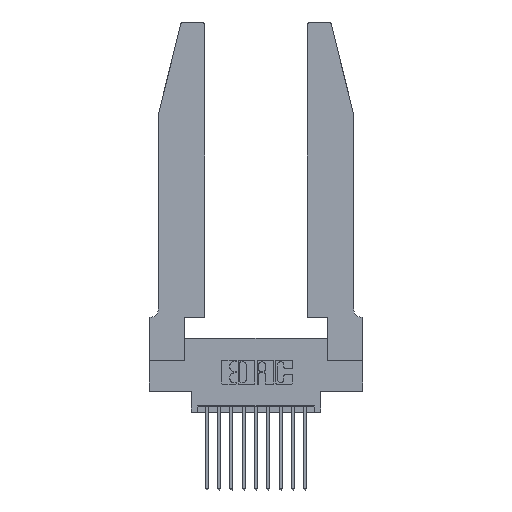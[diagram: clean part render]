
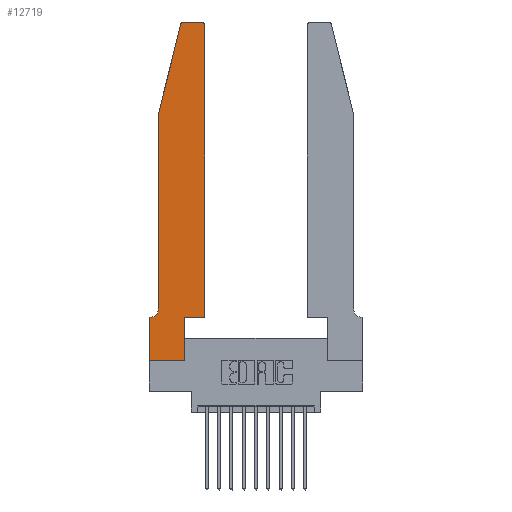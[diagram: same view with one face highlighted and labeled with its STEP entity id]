
A CAD part, top view. The second image highlights one B-rep face of the part: STEP entity #12719.
In plain terms, the highlighted planar face has unit normal (0, 0, 1).
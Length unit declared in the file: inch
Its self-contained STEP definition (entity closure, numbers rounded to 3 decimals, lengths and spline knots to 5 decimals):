
#7 = VERTEX_POINT ( 'NONE', #5723 ) ;
#8 = ORIENTED_EDGE ( 'NONE', *, *, #6700, .T. ) ;
#240 = VECTOR ( 'NONE', #7956, 39.37008 ) ;
#513 = EDGE_CURVE ( 'NONE', #15229, #9144, #12579, .T. ) ;
#574 = CARTESIAN_POINT ( 'NONE',  ( 0.0755, 2., 0.37 ) ) ;
#583 = DIRECTION ( 'NONE',  ( 0., -1., 0. ) ) ;
#691 = EDGE_CURVE ( 'NONE', #2168, #7, #15413, .T. ) ;
#982 = CARTESIAN_POINT ( 'NONE',  ( 0.2865, 0.35, 0.37 ) ) ;
#1098 = CARTESIAN_POINT ( 'NONE',  ( 0.0755, 2., 0.37 ) ) ;
#1359 = VERTEX_POINT ( 'NONE', #3333 ) ;
#1616 = CARTESIAN_POINT ( 'NONE',  ( 0.4205, 2.72, 0.37 ) ) ;
#1699 = AXIS2_PLACEMENT_3D ( 'NONE', #1616, #13079, #7651 ) ;
#1949 = VERTEX_POINT ( 'NONE', #6320 ) ;
#2044 = CARTESIAN_POINT ( 'NONE',  ( 0.25487, 2.72718, 0.37 ) ) ;
#2168 = VERTEX_POINT ( 'NONE', #1098 ) ;
#2237 = DIRECTION ( 'NONE',  ( 0., 1., 0. ) ) ;
#2450 = CIRCLE ( 'NONE', #9454, 0.07 ) ;
#2616 = EDGE_CURVE ( 'NONE', #7, #9449, #2450, .T. ) ;
#2833 = VECTOR ( 'NONE', #2237, 39.37008 ) ;
#2971 = LINE ( 'NONE', #574, #12262 ) ;
#3333 = CARTESIAN_POINT ( 'NONE',  ( 0.4505, 2.72, 0.37 ) ) ;
#3391 = DIRECTION ( 'NONE',  ( 0., -1., 0. ) ) ;
#3538 = DIRECTION ( 'NONE',  ( 1., 0., 0. ) ) ;
#3637 = ORIENTED_EDGE ( 'NONE', *, *, #513, .T. ) ;
#3821 = FACE_OUTER_BOUND ( 'NONE', #3955, .T. ) ;
#3896 = CARTESIAN_POINT ( 'NONE',  ( 0.4505, 0.35, 0.37 ) ) ;
#3955 = EDGE_LOOP ( 'NONE', ( #10260, #14489, #6362, #4399, #6009, #8, #13393, #8602, #4469, #3637, #14620, #6218 ) ) ;
#4399 = ORIENTED_EDGE ( 'NONE', *, *, #691, .T. ) ;
#4469 = ORIENTED_EDGE ( 'NONE', *, *, #11685, .T. ) ;
#4713 = VERTEX_POINT ( 'NONE', #11593 ) ;
#4882 = CARTESIAN_POINT ( 'NONE',  ( 0.284, 2.72, 0.37 ) ) ;
#4922 = VECTOR ( 'NONE', #11745, 39.37008 ) ;
#5212 = CARTESIAN_POINT ( 'NONE',  ( 0.4205, 2.75, 0.37 ) ) ;
#5274 = VECTOR ( 'NONE', #3391, 39.37008 ) ;
#5364 = CARTESIAN_POINT ( 'NONE',  ( 0.2605, 2.75, 0.37 ) ) ;
#5405 = CARTESIAN_POINT ( 'NONE',  ( 0.0755, 0.35, 0.37 ) ) ;
#5448 = VERTEX_POINT ( 'NONE', #5212 ) ;
#5534 = LINE ( 'NONE', #11857, #11281 ) ;
#5586 = DIRECTION ( 'NONE',  ( 0., 0., -1. ) ) ;
#5631 = CARTESIAN_POINT ( 'NONE',  ( 0., 0.35, 0.37 ) ) ;
#5656 = CARTESIAN_POINT ( 'NONE',  ( 0., 0., 0.37 ) ) ;
#5712 = LINE ( 'NONE', #8702, #13417 ) ;
#5723 = CARTESIAN_POINT ( 'NONE',  ( 0.0755, 0.42, 0.37 ) ) ;
#5975 = DIRECTION ( 'NONE',  ( 1., 0., 0. ) ) ;
#6009 = ORIENTED_EDGE ( 'NONE', *, *, #2616, .T. ) ;
#6083 = VECTOR ( 'NONE', #9026, 39.37008 ) ;
#6140 = PLANE ( 'NONE',  #15757 ) ;
#6218 = ORIENTED_EDGE ( 'NONE', *, *, #11066, .T. ) ;
#6320 = CARTESIAN_POINT ( 'NONE',  ( 0.2865, 0., 0.37 ) ) ;
#6362 = ORIENTED_EDGE ( 'NONE', *, *, #7263, .T. ) ;
#6386 = CARTESIAN_POINT ( 'NONE',  ( 0.0055, 0.35, 0.37 ) ) ;
#6700 = EDGE_CURVE ( 'NONE', #9449, #8165, #10301, .T. ) ;
#7263 = EDGE_CURVE ( 'NONE', #12573, #2168, #2971, .T. ) ;
#7651 = DIRECTION ( 'NONE',  ( 1., 0., 0. ) ) ;
#7901 = EDGE_CURVE ( 'NONE', #9144, #1359, #5534, .T. ) ;
#7956 = DIRECTION ( 'NONE',  ( -1., 0., 0. ) ) ;
#8165 = VERTEX_POINT ( 'NONE', #5631 ) ;
#8236 = CIRCLE ( 'NONE', #1699, 0.03 ) ;
#8563 = CARTESIAN_POINT ( 'NONE',  ( 0.0755, 2., 0.37 ) ) ;
#8584 = CIRCLE ( 'NONE', #14884, 0.03 ) ;
#8602 = ORIENTED_EDGE ( 'NONE', *, *, #9810, .T. ) ;
#8636 = CARTESIAN_POINT ( 'NONE',  ( 0., 0.35, 0.37 ) ) ;
#8702 = CARTESIAN_POINT ( 'NONE',  ( 0., 0., 0.37 ) ) ;
#8987 = CARTESIAN_POINT ( 'NONE',  ( 0.2865, 0.35, 0.37 ) ) ;
#9026 = DIRECTION ( 'NONE',  ( 1., 0., 0. ) ) ;
#9144 = VERTEX_POINT ( 'NONE', #11086 ) ;
#9381 = VERTEX_POINT ( 'NONE', #5656 ) ;
#9449 = VERTEX_POINT ( 'NONE', #6386 ) ;
#9454 = AXIS2_PLACEMENT_3D ( 'NONE', #15761, #5586, #10548 ) ;
#9810 = EDGE_CURVE ( 'NONE', #9381, #1949, #5712, .T. ) ;
#9909 = EDGE_CURVE ( 'NONE', #5448, #4713, #16037, .T. ) ;
#10146 = LINE ( 'NONE', #15778, #11924 ) ;
#10260 = ORIENTED_EDGE ( 'NONE', *, *, #9909, .T. ) ;
#10301 = LINE ( 'NONE', #5405, #240 ) ;
#10548 = DIRECTION ( 'NONE',  ( -1., 0., 0. ) ) ;
#11066 = EDGE_CURVE ( 'NONE', #1359, #5448, #8236, .T. ) ;
#11086 = CARTESIAN_POINT ( 'NONE',  ( 0.4505, 0.35, 0.37 ) ) ;
#11281 = VECTOR ( 'NONE', #13149, 39.37008 ) ;
#11593 = CARTESIAN_POINT ( 'NONE',  ( 0.284, 2.75, 0.37 ) ) ;
#11685 = EDGE_CURVE ( 'NONE', #1949, #15229, #15157, .T. ) ;
#11745 = DIRECTION ( 'NONE',  ( -1., 0., 0. ) ) ;
#11857 = CARTESIAN_POINT ( 'NONE',  ( 0.4505, 0.35, 0.37 ) ) ;
#11924 = VECTOR ( 'NONE', #583, 39.37008 ) ;
#12262 = VECTOR ( 'NONE', #15643, 39.37008 ) ;
#12382 = EDGE_CURVE ( 'NONE', #8165, #9381, #10146, .T. ) ;
#12573 = VERTEX_POINT ( 'NONE', #2044 ) ;
#12579 = LINE ( 'NONE', #3896, #6083 ) ;
#12653 = EDGE_CURVE ( 'NONE', #4713, #12573, #8584, .T. ) ;
#12719 = ADVANCED_FACE ( 'NONE', ( #3821 ), #6140, .T. ) ;
#13079 = DIRECTION ( 'NONE',  ( 0., 0., 1. ) ) ;
#13149 = DIRECTION ( 'NONE',  ( 0., 1., 0. ) ) ;
#13393 = ORIENTED_EDGE ( 'NONE', *, *, #12382, .T. ) ;
#13417 = VECTOR ( 'NONE', #13620, 39.37008 ) ;
#13620 = DIRECTION ( 'NONE',  ( 1., 0., 0. ) ) ;
#13715 = DIRECTION ( 'NONE',  ( 0., 0., 1. ) ) ;
#14489 = ORIENTED_EDGE ( 'NONE', *, *, #12653, .T. ) ;
#14620 = ORIENTED_EDGE ( 'NONE', *, *, #7901, .T. ) ;
#14884 = AXIS2_PLACEMENT_3D ( 'NONE', #4882, #13715, #3538 ) ;
#15016 = DIRECTION ( 'NONE',  ( 0., 0., 1. ) ) ;
#15157 = LINE ( 'NONE', #982, #2833 ) ;
#15229 = VERTEX_POINT ( 'NONE', #8987 ) ;
#15413 = LINE ( 'NONE', #8563, #5274 ) ;
#15643 = DIRECTION ( 'NONE',  ( -0.239, -0.971, 0. ) ) ;
#15757 = AXIS2_PLACEMENT_3D ( 'NONE', #8636, #15016, #5975 ) ;
#15761 = CARTESIAN_POINT ( 'NONE',  ( 0.0055, 0.42, 0.37 ) ) ;
#15778 = CARTESIAN_POINT ( 'NONE',  ( 0., 0., 0.37 ) ) ;
#16037 = LINE ( 'NONE', #5364, #4922 ) ;
